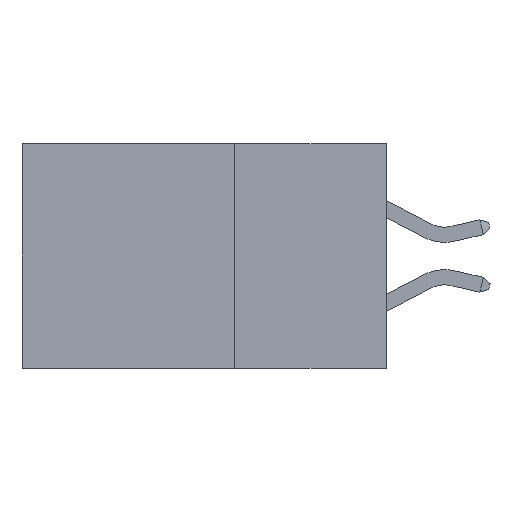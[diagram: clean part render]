
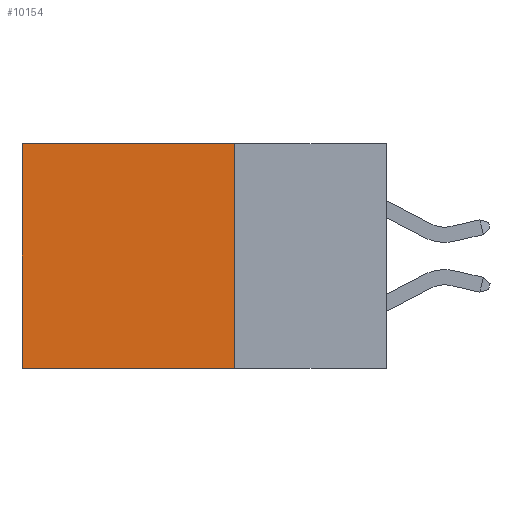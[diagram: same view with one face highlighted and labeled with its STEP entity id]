
A CAD part, left-side view. The second image highlights one B-rep face of the part: STEP entity #10154.
In plain terms, the highlighted planar face has unit normal (-1, 0, 0).
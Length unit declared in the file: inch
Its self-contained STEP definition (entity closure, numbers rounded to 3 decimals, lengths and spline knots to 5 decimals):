
#68 = ORIENTED_EDGE ( 'NONE', *, *, #3018, .T. ) ;
#446 = EDGE_CURVE ( 'NONE', #7758, #12851, #8017, .T. ) ;
#1484 = EDGE_CURVE ( 'NONE', #12117, #7758, #9686, .T. ) ;
#2220 = CARTESIAN_POINT ( 'NONE',  ( 0.298, 0.25, 0. ) ) ;
#2423 = DIRECTION ( 'NONE',  ( 0., 0., -1. ) ) ;
#2742 = CARTESIAN_POINT ( 'NONE',  ( 0.298, 0.6, -0.37 ) ) ;
#3018 = EDGE_CURVE ( 'NONE', #12117, #4262, #4580, .T. ) ;
#3936 = CARTESIAN_POINT ( 'NONE',  ( 0.298, 0.25, 0. ) ) ;
#4119 = CARTESIAN_POINT ( 'NONE',  ( 0.298, 0.25, -0.37 ) ) ;
#4148 = FACE_OUTER_BOUND ( 'NONE', #7615, .T. ) ;
#4262 = VERTEX_POINT ( 'NONE', #6744 ) ;
#4580 = LINE ( 'NONE', #5474, #6781 ) ;
#5185 = PLANE ( 'NONE',  #8355 ) ;
#5463 = ORIENTED_EDGE ( 'NONE', *, *, #8466, .T. ) ;
#5474 = CARTESIAN_POINT ( 'NONE',  ( 0.298, 0.25, 0. ) ) ;
#5573 = ORIENTED_EDGE ( 'NONE', *, *, #446, .F. ) ;
#6122 = VECTOR ( 'NONE', #13017, 39.37008 ) ;
#6744 = CARTESIAN_POINT ( 'NONE',  ( 0.298, 0.6, 0. ) ) ;
#6781 = VECTOR ( 'NONE', #9860, 39.37008 ) ;
#6833 = VECTOR ( 'NONE', #2423, 39.37008 ) ;
#7002 = VECTOR ( 'NONE', #10822, 39.37008 ) ;
#7615 = EDGE_LOOP ( 'NONE', ( #5463, #5573, #7911, #68 ) ) ;
#7742 = CARTESIAN_POINT ( 'NONE',  ( 0.298, 0.25, 0. ) ) ;
#7755 = CARTESIAN_POINT ( 'NONE',  ( 0.298, 0.25, -0.37 ) ) ;
#7758 = VERTEX_POINT ( 'NONE', #4119 ) ;
#7911 = ORIENTED_EDGE ( 'NONE', *, *, #1484, .F. ) ;
#8017 = LINE ( 'NONE', #7755, #7002 ) ;
#8355 = AXIS2_PLACEMENT_3D ( 'NONE', #2220, #10302, #8603 ) ;
#8466 = EDGE_CURVE ( 'NONE', #4262, #12851, #8975, .T. ) ;
#8603 = DIRECTION ( 'NONE',  ( 0., 0., -1. ) ) ;
#8975 = LINE ( 'NONE', #9525, #6122 ) ;
#9525 = CARTESIAN_POINT ( 'NONE',  ( 0.298, 0.6, 0. ) ) ;
#9686 = LINE ( 'NONE', #7742, #6833 ) ;
#9860 = DIRECTION ( 'NONE',  ( 0., 1., 0. ) ) ;
#10154 = ADVANCED_FACE ( 'NONE', ( #4148 ), #5185, .F. ) ;
#10302 = DIRECTION ( 'NONE',  ( 1., 0., 0. ) ) ;
#10822 = DIRECTION ( 'NONE',  ( 0., 1., 0. ) ) ;
#12117 = VERTEX_POINT ( 'NONE', #3936 ) ;
#12851 = VERTEX_POINT ( 'NONE', #2742 ) ;
#13017 = DIRECTION ( 'NONE',  ( 0., 0., -1. ) ) ;
